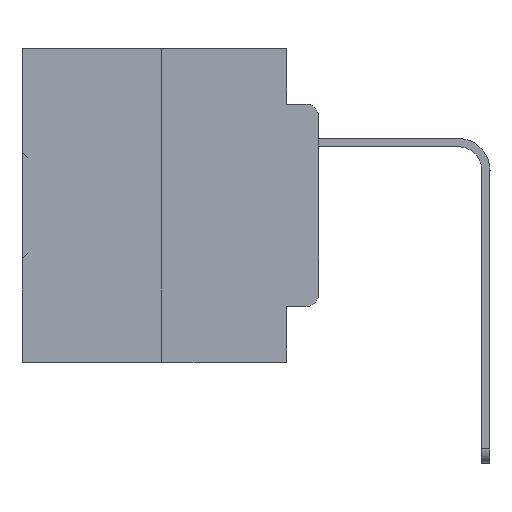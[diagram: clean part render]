
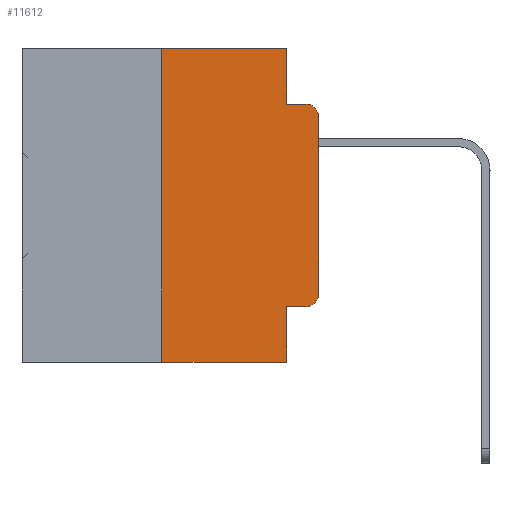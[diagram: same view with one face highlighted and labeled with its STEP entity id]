
A CAD part, left-side view. The second image highlights one B-rep face of the part: STEP entity #11612.
In plain terms, the highlighted planar face has unit normal (-1, 0, 0).
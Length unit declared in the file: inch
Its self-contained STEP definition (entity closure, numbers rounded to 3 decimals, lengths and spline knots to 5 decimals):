
#2759 = DIRECTION ( 'NONE',  ( -1., 0., 0. ) ) ;
#3412 = LINE ( 'NONE', #7613, #8821 ) ;
#3586 = LINE ( 'NONE', #6938, #23653 ) ;
#5879 = EDGE_CURVE ( 'NONE', #32038, #15792, #3412, .T. ) ;
#6178 = VERTEX_POINT ( 'NONE', #14979 ) ;
#6189 = ORIENTED_EDGE ( 'NONE', *, *, #9943, .T. ) ;
#6494 = DIRECTION ( 'NONE',  ( 1., 0., 0. ) ) ;
#6531 = LINE ( 'NONE', #9785, #33290 ) ;
#6576 = DIRECTION ( 'NONE',  ( 0., 0., -1. ) ) ;
#6914 = VECTOR ( 'NONE', #31118, 39.37008 ) ;
#6938 = CARTESIAN_POINT ( 'NONE',  ( 0., 0.051, 0. ) ) ;
#7412 = VERTEX_POINT ( 'NONE', #23424 ) ;
#7613 = CARTESIAN_POINT ( 'NONE',  ( 0., 0.051, -0.4115 ) ) ;
#8821 = VECTOR ( 'NONE', #28523, 39.37008 ) ;
#8863 = DIRECTION ( 'NONE',  ( 0., 0., 1. ) ) ;
#8898 = FACE_OUTER_BOUND ( 'NONE', #32535, .T. ) ;
#8912 = LINE ( 'NONE', #33145, #21072 ) ;
#8943 = ORIENTED_EDGE ( 'NONE', *, *, #34298, .T. ) ;
#9785 = CARTESIAN_POINT ( 'NONE',  ( 0., 0.473, -0.5 ) ) ;
#9943 = EDGE_CURVE ( 'NONE', #33331, #6178, #6531, .T. ) ;
#10397 = EDGE_CURVE ( 'NONE', #10445, #30232, #3586, .T. ) ;
#10445 = VERTEX_POINT ( 'NONE', #20291 ) ;
#10531 = EDGE_CURVE ( 'NONE', #32038, #6178, #28232, .T. ) ;
#11209 = VECTOR ( 'NONE', #25355, 39.37008 ) ;
#11612 = ADVANCED_FACE ( 'NONE', ( #8898 ), #22291, .F. ) ;
#11915 = CIRCLE ( 'NONE', #16100, 0.02 ) ;
#12330 = CIRCLE ( 'NONE', #30520, 0.02 ) ;
#12430 = CARTESIAN_POINT ( 'NONE',  ( 0., 0.051, 0. ) ) ;
#14169 = ORIENTED_EDGE ( 'NONE', *, *, #15463, .F. ) ;
#14303 = VERTEX_POINT ( 'NONE', #21708 ) ;
#14979 = CARTESIAN_POINT ( 'NONE',  ( 0., 0.051, -0.5 ) ) ;
#15463 = EDGE_CURVE ( 'NONE', #33331, #22603, #24584, .T. ) ;
#15620 = CARTESIAN_POINT ( 'NONE',  ( 0., 0.051, -0.0885 ) ) ;
#15792 = VERTEX_POINT ( 'NONE', #19018 ) ;
#16100 = AXIS2_PLACEMENT_3D ( 'NONE', #21590, #2759, #27046 ) ;
#17398 = CARTESIAN_POINT ( 'NONE',  ( 0., 0.473, 0. ) ) ;
#17653 = CARTESIAN_POINT ( 'NONE',  ( 0., 0.25, 0. ) ) ;
#18743 = ORIENTED_EDGE ( 'NONE', *, *, #10397, .F. ) ;
#19018 = CARTESIAN_POINT ( 'NONE',  ( 0., 0.02, -0.4115 ) ) ;
#19152 = CARTESIAN_POINT ( 'NONE',  ( 0., 0.02, -0.0885 ) ) ;
#19463 = LINE ( 'NONE', #20532, #26966 ) ;
#20291 = CARTESIAN_POINT ( 'NONE',  ( 0., 0.051, 0. ) ) ;
#20532 = CARTESIAN_POINT ( 'NONE',  ( 0., 0.051, -0.0885 ) ) ;
#21072 = VECTOR ( 'NONE', #8863, 39.37008 ) ;
#21590 = CARTESIAN_POINT ( 'NONE',  ( 0., 0.02, -0.1085 ) ) ;
#21708 = CARTESIAN_POINT ( 'NONE',  ( 0., 0., -0.3915 ) ) ;
#21921 = ORIENTED_EDGE ( 'NONE', *, *, #22019, .F. ) ;
#22019 = EDGE_CURVE ( 'NONE', #30232, #25518, #19463, .T. ) ;
#22291 = PLANE ( 'NONE',  #34512 ) ;
#22603 = VERTEX_POINT ( 'NONE', #25356 ) ;
#23117 = EDGE_CURVE ( 'NONE', #14303, #7412, #8912, .T. ) ;
#23424 = CARTESIAN_POINT ( 'NONE',  ( 0., 0., -0.1085 ) ) ;
#23653 = VECTOR ( 'NONE', #6576, 39.37008 ) ;
#24084 = DIRECTION ( 'NONE',  ( 0., 0., -1. ) ) ;
#24584 = LINE ( 'NONE', #17653, #11209 ) ;
#25355 = DIRECTION ( 'NONE',  ( 0., 0., 1. ) ) ;
#25356 = CARTESIAN_POINT ( 'NONE',  ( 0., 0.25, 0. ) ) ;
#25518 = VERTEX_POINT ( 'NONE', #19152 ) ;
#26427 = ORIENTED_EDGE ( 'NONE', *, *, #32952, .F. ) ;
#26966 = VECTOR ( 'NONE', #34044, 39.37008 ) ;
#27046 = DIRECTION ( 'NONE',  ( 0., 0., -1. ) ) ;
#27147 = CARTESIAN_POINT ( 'NONE',  ( 0., 0.25, -0.5 ) ) ;
#27776 = CARTESIAN_POINT ( 'NONE',  ( 0., 0.473, 0. ) ) ;
#27813 = ORIENTED_EDGE ( 'NONE', *, *, #10531, .F. ) ;
#28232 = LINE ( 'NONE', #12430, #6914 ) ;
#28523 = DIRECTION ( 'NONE',  ( 0., -1., 0. ) ) ;
#29427 = ORIENTED_EDGE ( 'NONE', *, *, #30268, .T. ) ;
#29535 = CARTESIAN_POINT ( 'NONE',  ( 0., 0.051, -0.4115 ) ) ;
#30135 = ORIENTED_EDGE ( 'NONE', *, *, #5879, .T. ) ;
#30232 = VERTEX_POINT ( 'NONE', #15620 ) ;
#30268 = EDGE_CURVE ( 'NONE', #7412, #25518, #11915, .T. ) ;
#30471 = DIRECTION ( 'NONE',  ( 0., -1., 0. ) ) ;
#30520 = AXIS2_PLACEMENT_3D ( 'NONE', #32115, #31646, #24084 ) ;
#30600 = ORIENTED_EDGE ( 'NONE', *, *, #23117, .T. ) ;
#31118 = DIRECTION ( 'NONE',  ( 0., 0., -1. ) ) ;
#31333 = LINE ( 'NONE', #27776, #32567 ) ;
#31646 = DIRECTION ( 'NONE',  ( -1., 0., 0. ) ) ;
#31820 = DIRECTION ( 'NONE',  ( 0., -1., 0. ) ) ;
#32038 = VERTEX_POINT ( 'NONE', #29535 ) ;
#32115 = CARTESIAN_POINT ( 'NONE',  ( 0., 0.02, -0.3915 ) ) ;
#32535 = EDGE_LOOP ( 'NONE', ( #30600, #29427, #21921, #18743, #26427, #14169, #6189, #27813, #30135, #8943 ) ) ;
#32567 = VECTOR ( 'NONE', #30471, 39.37008 ) ;
#32894 = DIRECTION ( 'NONE',  ( 0., 0., -1. ) ) ;
#32952 = EDGE_CURVE ( 'NONE', #22603, #10445, #31333, .T. ) ;
#33145 = CARTESIAN_POINT ( 'NONE',  ( 0., 0., 0. ) ) ;
#33290 = VECTOR ( 'NONE', #31820, 39.37008 ) ;
#33331 = VERTEX_POINT ( 'NONE', #27147 ) ;
#34044 = DIRECTION ( 'NONE',  ( 0., -1., 0. ) ) ;
#34298 = EDGE_CURVE ( 'NONE', #15792, #14303, #12330, .T. ) ;
#34512 = AXIS2_PLACEMENT_3D ( 'NONE', #17398, #6494, #32894 ) ;
